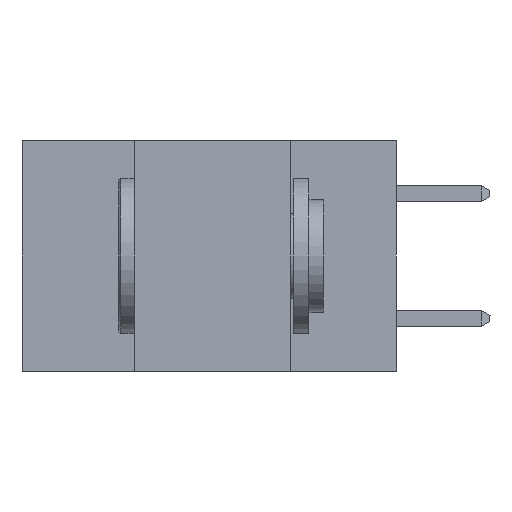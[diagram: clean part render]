
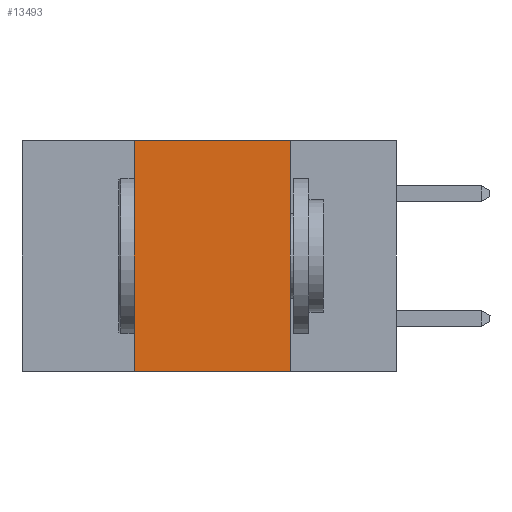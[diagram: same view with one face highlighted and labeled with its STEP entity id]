
A CAD part, left-side view. The second image highlights one B-rep face of the part: STEP entity #13493.
In plain terms, the highlighted planar face has unit normal (-1, 0, 0).
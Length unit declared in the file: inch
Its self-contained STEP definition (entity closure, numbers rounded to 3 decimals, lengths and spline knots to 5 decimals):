
#22 = DIRECTION ( 'NONE',  ( 0., 0., -1. ) ) ;
#511 = DIRECTION ( 'NONE',  ( 0., 0., -1. ) ) ;
#1007 = CARTESIAN_POINT ( 'NONE',  ( 0., 0.6, 0. ) ) ;
#1140 = DIRECTION ( 'NONE',  ( 1., 0., 0. ) ) ;
#1952 = LINE ( 'NONE', #5805, #8322 ) ;
#2038 = LINE ( 'NONE', #8115, #10861 ) ;
#2071 = EDGE_CURVE ( 'NONE', #5964, #4106, #1952, .T. ) ;
#2294 = ORIENTED_EDGE ( 'NONE', *, *, #10479, .T. ) ;
#2567 = FACE_OUTER_BOUND ( 'NONE', #14180, .T. ) ;
#3425 = VECTOR ( 'NONE', #4614, 39.37008 ) ;
#4106 = VERTEX_POINT ( 'NONE', #16539 ) ;
#4614 = DIRECTION ( 'NONE',  ( 0., 0., 1. ) ) ;
#4825 = PLANE ( 'NONE',  #14980 ) ;
#5507 = DIRECTION ( 'NONE',  ( 0., -1., 0. ) ) ;
#5805 = CARTESIAN_POINT ( 'NONE',  ( 0., 0.17, 0. ) ) ;
#5964 = VERTEX_POINT ( 'NONE', #16527 ) ;
#6123 = CARTESIAN_POINT ( 'NONE',  ( 0., 0.42, -0.37 ) ) ;
#6433 = CARTESIAN_POINT ( 'NONE',  ( 0., 0.42, 0. ) ) ;
#7028 = CARTESIAN_POINT ( 'NONE',  ( 0., 0.42, 0. ) ) ;
#8115 = CARTESIAN_POINT ( 'NONE',  ( 0., 0.6, -0.37 ) ) ;
#8322 = VECTOR ( 'NONE', #511, 39.37008 ) ;
#8547 = VERTEX_POINT ( 'NONE', #6123 ) ;
#9350 = EDGE_CURVE ( 'NONE', #8547, #13537, #10268, .T. ) ;
#9709 = LINE ( 'NONE', #1007, #11723 ) ;
#10268 = LINE ( 'NONE', #7028, #3425 ) ;
#10479 = EDGE_CURVE ( 'NONE', #8547, #4106, #2038, .T. ) ;
#10494 = ORIENTED_EDGE ( 'NONE', *, *, #9350, .F. ) ;
#10861 = VECTOR ( 'NONE', #5507, 39.37008 ) ;
#11653 = ORIENTED_EDGE ( 'NONE', *, *, #15276, .F. ) ;
#11704 = DIRECTION ( 'NONE',  ( 0., -1., 0. ) ) ;
#11723 = VECTOR ( 'NONE', #11704, 39.37008 ) ;
#13493 = ADVANCED_FACE ( 'NONE', ( #2567 ), #4825, .F. ) ;
#13537 = VERTEX_POINT ( 'NONE', #6433 ) ;
#13807 = ORIENTED_EDGE ( 'NONE', *, *, #2071, .F. ) ;
#13818 = CARTESIAN_POINT ( 'NONE',  ( 0., 0.6, 0. ) ) ;
#14180 = EDGE_LOOP ( 'NONE', ( #13807, #11653, #10494, #2294 ) ) ;
#14980 = AXIS2_PLACEMENT_3D ( 'NONE', #13818, #1140, #22 ) ;
#15276 = EDGE_CURVE ( 'NONE', #13537, #5964, #9709, .T. ) ;
#16527 = CARTESIAN_POINT ( 'NONE',  ( 0., 0.17, 0. ) ) ;
#16539 = CARTESIAN_POINT ( 'NONE',  ( 0., 0.17, -0.37 ) ) ;
